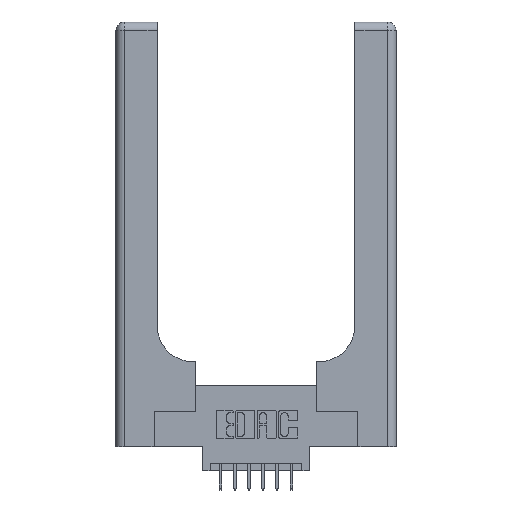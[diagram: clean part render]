
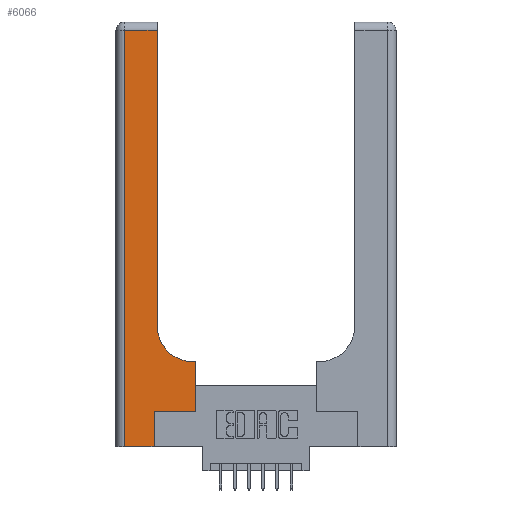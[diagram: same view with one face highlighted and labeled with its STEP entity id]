
A CAD part, top view. The second image highlights one B-rep face of the part: STEP entity #6066.
In plain terms, the highlighted planar face has unit normal (0, 0, 1).
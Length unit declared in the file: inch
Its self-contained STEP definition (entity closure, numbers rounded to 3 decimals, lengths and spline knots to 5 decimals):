
#48 = EDGE_CURVE ( 'NONE', #9242, #4076, #12172, .T. ) ;
#200 = EDGE_CURVE ( 'NONE', #14212, #9768, #14765, .T. ) ;
#484 = AXIS2_PLACEMENT_3D ( 'NONE', #8404, #1551, #4899 ) ;
#487 = DIRECTION ( 'NONE',  ( 0., 1., 0. ) ) ;
#495 = CIRCLE ( 'NONE', #484, 0.25 ) ;
#693 = VECTOR ( 'NONE', #10152, 39.37008 ) ;
#845 = VECTOR ( 'NONE', #4369, 39.37008 ) ;
#1013 = EDGE_LOOP ( 'NONE', ( #11691, #5049, #13098, #2992, #9785, #3882, #1834, #3885, #13010 ) ) ;
#1145 = VECTOR ( 'NONE', #4562, 39.37008 ) ;
#1169 = DIRECTION ( 'NONE',  ( 1., 0., 0. ) ) ;
#1328 = CARTESIAN_POINT ( 'NONE',  ( 0.06, 0., 0.37 ) ) ;
#1551 = DIRECTION ( 'NONE',  ( 0., 0., -1. ) ) ;
#1834 = ORIENTED_EDGE ( 'NONE', *, *, #4489, .T. ) ;
#2606 = AXIS2_PLACEMENT_3D ( 'NONE', #8985, #7860, #6342 ) ;
#2992 = ORIENTED_EDGE ( 'NONE', *, *, #200, .T. ) ;
#3078 = LINE ( 'NONE', #9908, #8096 ) ;
#3232 = CARTESIAN_POINT ( 'NONE',  ( 0.2915, 0.6, 0.37 ) ) ;
#3311 = LINE ( 'NONE', #3232, #14437 ) ;
#3882 = ORIENTED_EDGE ( 'NONE', *, *, #10252, .T. ) ;
#3885 = ORIENTED_EDGE ( 'NONE', *, *, #5732, .T. ) ;
#3995 = EDGE_CURVE ( 'NONE', #4076, #14212, #10174, .T. ) ;
#4076 = VERTEX_POINT ( 'NONE', #5996 ) ;
#4369 = DIRECTION ( 'NONE',  ( 1., 0., 0. ) ) ;
#4489 = EDGE_CURVE ( 'NONE', #14633, #14446, #7387, .T. ) ;
#4562 = DIRECTION ( 'NONE',  ( 0., -1., 0. ) ) ;
#4897 = CARTESIAN_POINT ( 'NONE',  ( 0.2915, 2.94, 0.37 ) ) ;
#4899 = DIRECTION ( 'NONE',  ( 1., 0., 0. ) ) ;
#5049 = ORIENTED_EDGE ( 'NONE', *, *, #48, .T. ) ;
#5609 = CARTESIAN_POINT ( 'NONE',  ( 0.5415, 0.6, 0.37 ) ) ;
#5732 = EDGE_CURVE ( 'NONE', #14446, #5735, #3311, .T. ) ;
#5735 = VERTEX_POINT ( 'NONE', #5609 ) ;
#5760 = CARTESIAN_POINT ( 'NONE',  ( 0.269, 0., 0.37 ) ) ;
#5996 = CARTESIAN_POINT ( 'NONE',  ( 0.06, 2.94, 0.37 ) ) ;
#6066 = ADVANCED_FACE ( 'NONE', ( #12102 ), #10268, .F. ) ;
#6145 = VERTEX_POINT ( 'NONE', #6157 ) ;
#6157 = CARTESIAN_POINT ( 'NONE',  ( 0.2915, 0.85, 0.37 ) ) ;
#6342 = DIRECTION ( 'NONE',  ( -1., 0., 0. ) ) ;
#6406 = VECTOR ( 'NONE', #12257, 39.37008 ) ;
#7354 = EDGE_CURVE ( 'NONE', #6145, #9242, #8869, .T. ) ;
#7387 = LINE ( 'NONE', #14323, #9820 ) ;
#7860 = DIRECTION ( 'NONE',  ( 0., 0., -1. ) ) ;
#8096 = VECTOR ( 'NONE', #8638, 39.37008 ) ;
#8404 = CARTESIAN_POINT ( 'NONE',  ( 0.5415, 0.85, 0.37 ) ) ;
#8638 = DIRECTION ( 'NONE',  ( 0., 1., 0. ) ) ;
#8869 = LINE ( 'NONE', #13490, #693 ) ;
#8985 = CARTESIAN_POINT ( 'NONE',  ( 0., 3., 0.37 ) ) ;
#9024 = LINE ( 'NONE', #11393, #10651 ) ;
#9242 = VERTEX_POINT ( 'NONE', #4897 ) ;
#9768 = VERTEX_POINT ( 'NONE', #5760 ) ;
#9785 = ORIENTED_EDGE ( 'NONE', *, *, #13311, .T. ) ;
#9820 = VECTOR ( 'NONE', #487, 39.37008 ) ;
#9903 = EDGE_CURVE ( 'NONE', #5735, #6145, #495, .T. ) ;
#9908 = CARTESIAN_POINT ( 'NONE',  ( 0.269, 0., 0.37 ) ) ;
#10099 = CARTESIAN_POINT ( 'NONE',  ( 0.06, 3., 0.37 ) ) ;
#10152 = DIRECTION ( 'NONE',  ( 0., 1., 0. ) ) ;
#10174 = LINE ( 'NONE', #10099, #1145 ) ;
#10252 = EDGE_CURVE ( 'NONE', #14510, #14633, #9024, .T. ) ;
#10268 = PLANE ( 'NONE',  #2606 ) ;
#10302 = CARTESIAN_POINT ( 'NONE',  ( 0.5585, 0.25, 0.37 ) ) ;
#10651 = VECTOR ( 'NONE', #1169, 39.37008 ) ;
#10786 = CARTESIAN_POINT ( 'NONE',  ( 0.5585, 0.6, 0.37 ) ) ;
#11393 = CARTESIAN_POINT ( 'NONE',  ( 0.269, 0.25, 0.37 ) ) ;
#11656 = CARTESIAN_POINT ( 'NONE',  ( 0., 0., 0.37 ) ) ;
#11691 = ORIENTED_EDGE ( 'NONE', *, *, #7354, .T. ) ;
#12102 = FACE_OUTER_BOUND ( 'NONE', #1013, .T. ) ;
#12172 = LINE ( 'NONE', #14438, #6406 ) ;
#12257 = DIRECTION ( 'NONE',  ( -1., 0., 0. ) ) ;
#12537 = CARTESIAN_POINT ( 'NONE',  ( 0.269, 0.25, 0.37 ) ) ;
#13010 = ORIENTED_EDGE ( 'NONE', *, *, #9903, .T. ) ;
#13098 = ORIENTED_EDGE ( 'NONE', *, *, #3995, .T. ) ;
#13311 = EDGE_CURVE ( 'NONE', #9768, #14510, #3078, .T. ) ;
#13490 = CARTESIAN_POINT ( 'NONE',  ( 0.2915, 3., 0.37 ) ) ;
#14212 = VERTEX_POINT ( 'NONE', #1328 ) ;
#14323 = CARTESIAN_POINT ( 'NONE',  ( 0.5585, 0.25, 0.37 ) ) ;
#14437 = VECTOR ( 'NONE', #14781, 39.37008 ) ;
#14438 = CARTESIAN_POINT ( 'NONE',  ( 0., 2.94, 0.37 ) ) ;
#14446 = VERTEX_POINT ( 'NONE', #10786 ) ;
#14510 = VERTEX_POINT ( 'NONE', #12537 ) ;
#14633 = VERTEX_POINT ( 'NONE', #10302 ) ;
#14765 = LINE ( 'NONE', #11656, #845 ) ;
#14781 = DIRECTION ( 'NONE',  ( -1., 0., 0. ) ) ;
